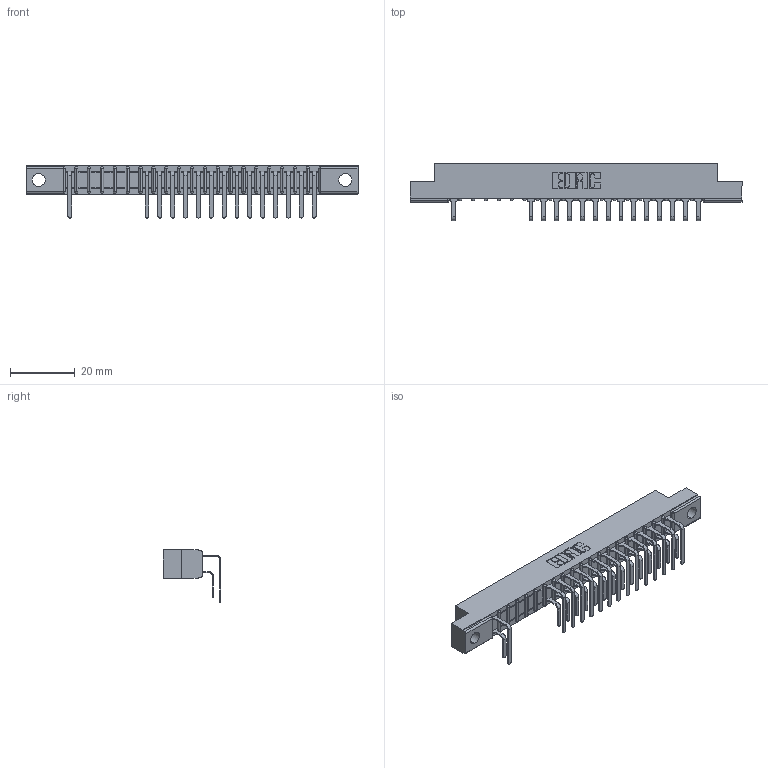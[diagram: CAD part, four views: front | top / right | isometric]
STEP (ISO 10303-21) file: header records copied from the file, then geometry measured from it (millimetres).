
FILE_DESCRIPTION (( 'STEP AP203' ), '1' );
FILE_NAME ('357-020-559-104.STEP', '2018-08-08T07:47:20', ( '' ), ( '' ), 'SwSTEP 2.0', 'SolidWorks 2016', '' );
FILE_SCHEMA (( 'CONFIG_CONTROL_DESIGN' ));
Length unit declared in the file: inch
Products named in the file (4): 357-020-559-104; 307 Part_.156 Dia Mounting Holes; 307-290-001_558 559 - 1 (Single); 307-290-001_559 - 2 (Single)
Assembly tree (31 placements, depth 2):
  357-020-559-104
    307 Part_.156 Dia Mounting Holes
    307-290-001_558 559 - 1 (Single)  x15
    307-290-001_559 - 2 (Single)  x15
Bounding box: 102.26 x 17.69 x 16.08 mm (x, y, z)
Volume: 6586.7 mm3; surface area: 11402 mm2
Topology: 31 solids, 31 shells, 1753 faces, 4939 edges, 3194 vertices
Faces by surface type: plane 1134, cylinder 577, sphere 42
Entity records: 22043 total; most frequent: CARTESIAN_POINT 3662, ORIENTED_EDGE 3634, DIRECTION 3577, EDGE_CURVE 1817, VECTOR 1391, LINE 1391, VERTEX_POINT 1178, AXIS2_PLACEMENT_3D 1093
